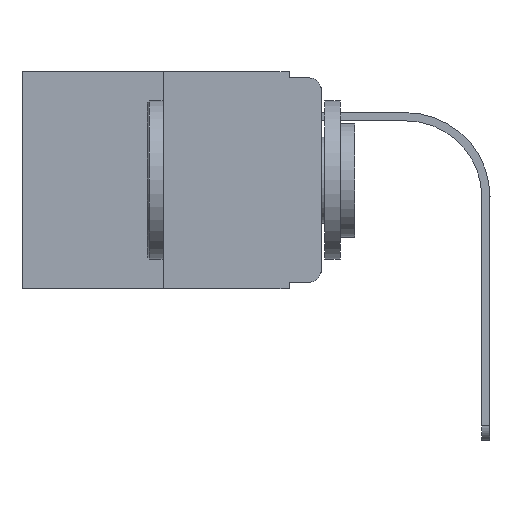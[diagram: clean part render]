
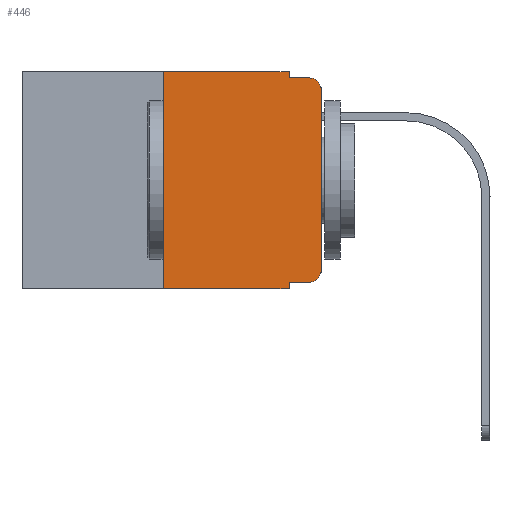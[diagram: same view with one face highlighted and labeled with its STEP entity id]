
A CAD part, left-side view. The second image highlights one B-rep face of the part: STEP entity #446.
In plain terms, the highlighted planar face has unit normal (-1, 0, 0).
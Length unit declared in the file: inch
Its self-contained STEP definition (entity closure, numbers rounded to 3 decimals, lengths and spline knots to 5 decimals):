
#70 = CIRCLE ( 'NONE', #8599, 0.02 ) ;
#167 = CARTESIAN_POINT ( 'NONE',  ( 0., 0.051, -0.01 ) ) ;
#170 = DIRECTION ( 'NONE',  ( -1., 0., 0. ) ) ;
#378 = CARTESIAN_POINT ( 'NONE',  ( 0., 0.473, 0. ) ) ;
#443 = VERTEX_POINT ( 'NONE', #7598 ) ;
#446 = ADVANCED_FACE ( 'NONE', ( #5929 ), #6590, .F. ) ;
#453 = DIRECTION ( 'NONE',  ( -1., 0., 0. ) ) ;
#575 = CARTESIAN_POINT ( 'NONE',  ( 0., 0.051, -0.343 ) ) ;
#637 = ORIENTED_EDGE ( 'NONE', *, *, #2398, .T. ) ;
#761 = EDGE_CURVE ( 'NONE', #2186, #443, #2042, .T. ) ;
#1385 = AXIS2_PLACEMENT_3D ( 'NONE', #9173, #170, #10749 ) ;
#1417 = CARTESIAN_POINT ( 'NONE',  ( 0., 0.25, -0.343 ) ) ;
#1520 = DIRECTION ( 'NONE',  ( 0., -1., 0. ) ) ;
#1544 = EDGE_CURVE ( 'NONE', #6409, #6714, #2971, .T. ) ;
#1589 = EDGE_LOOP ( 'NONE', ( #637, #8247, #5417, #9334, #9422, #5119, #8029, #5951, #1604, #4368 ) ) ;
#1604 = ORIENTED_EDGE ( 'NONE', *, *, #9402, .T. ) ;
#1634 = CARTESIAN_POINT ( 'NONE',  ( 0., 0.473, 0. ) ) ;
#2009 = CARTESIAN_POINT ( 'NONE',  ( 0., 0.051, 0. ) ) ;
#2042 = LINE ( 'NONE', #167, #7669 ) ;
#2082 = VECTOR ( 'NONE', #5662, 39.37008 ) ;
#2095 = VECTOR ( 'NONE', #1520, 39.37008 ) ;
#2110 = LINE ( 'NONE', #5325, #5553 ) ;
#2180 = LINE ( 'NONE', #3012, #2095 ) ;
#2186 = VERTEX_POINT ( 'NONE', #6053 ) ;
#2323 = CARTESIAN_POINT ( 'NONE',  ( 0., 0.051, 0. ) ) ;
#2398 = EDGE_CURVE ( 'NONE', #6714, #8966, #7943, .T. ) ;
#2554 = DIRECTION ( 'NONE',  ( 0., 0., 1. ) ) ;
#2668 = EDGE_CURVE ( 'NONE', #9132, #8607, #10073, .T. ) ;
#2971 = CIRCLE ( 'NONE', #1385, 0.02 ) ;
#3012 = CARTESIAN_POINT ( 'NONE',  ( 0., 0.473, -0.343 ) ) ;
#3018 = EDGE_CURVE ( 'NONE', #9859, #2186, #8878, .T. ) ;
#3308 = EDGE_CURVE ( 'NONE', #10294, #4684, #6876, .T. ) ;
#3467 = EDGE_CURVE ( 'NONE', #9132, #4684, #2180, .T. ) ;
#3662 = VECTOR ( 'NONE', #9560, 39.37008 ) ;
#4128 = DIRECTION ( 'NONE',  ( 0., 0., -1. ) ) ;
#4368 = ORIENTED_EDGE ( 'NONE', *, *, #1544, .T. ) ;
#4684 = VERTEX_POINT ( 'NONE', #575 ) ;
#5119 = ORIENTED_EDGE ( 'NONE', *, *, #2668, .F. ) ;
#5297 = CARTESIAN_POINT ( 'NONE',  ( 0., 0.051, 0. ) ) ;
#5325 = CARTESIAN_POINT ( 'NONE',  ( 0., 0.051, -0.333 ) ) ;
#5417 = ORIENTED_EDGE ( 'NONE', *, *, #761, .F. ) ;
#5553 = VECTOR ( 'NONE', #7751, 39.37008 ) ;
#5662 = DIRECTION ( 'NONE',  ( 0., 0., -1. ) ) ;
#5929 = FACE_OUTER_BOUND ( 'NONE', #1589, .T. ) ;
#5951 = ORIENTED_EDGE ( 'NONE', *, *, #3308, .F. ) ;
#6053 = CARTESIAN_POINT ( 'NONE',  ( 0., 0.051, -0.01 ) ) ;
#6409 = VERTEX_POINT ( 'NONE', #8992 ) ;
#6590 = PLANE ( 'NONE',  #7905 ) ;
#6611 = EDGE_CURVE ( 'NONE', #8966, #443, #70, .T. ) ;
#6714 = VERTEX_POINT ( 'NONE', #8683 ) ;
#6876 = LINE ( 'NONE', #2009, #3662 ) ;
#6948 = VECTOR ( 'NONE', #2554, 39.37008 ) ;
#6988 = VECTOR ( 'NONE', #8813, 39.37008 ) ;
#7397 = DIRECTION ( 'NONE',  ( 1., 0., 0. ) ) ;
#7598 = CARTESIAN_POINT ( 'NONE',  ( 0., 0.02, -0.01 ) ) ;
#7669 = VECTOR ( 'NONE', #8662, 39.37008 ) ;
#7751 = DIRECTION ( 'NONE',  ( 0., -1., 0. ) ) ;
#7905 = AXIS2_PLACEMENT_3D ( 'NONE', #1634, #7397, #4128 ) ;
#7908 = CARTESIAN_POINT ( 'NONE',  ( 0., 0.051, -0.333 ) ) ;
#7943 = LINE ( 'NONE', #10383, #6988 ) ;
#8029 = ORIENTED_EDGE ( 'NONE', *, *, #3467, .T. ) ;
#8247 = ORIENTED_EDGE ( 'NONE', *, *, #6611, .T. ) ;
#8316 = CARTESIAN_POINT ( 'NONE',  ( 0., 0., -0.03 ) ) ;
#8523 = DIRECTION ( 'NONE',  ( 0., 0., -1. ) ) ;
#8541 = VECTOR ( 'NONE', #9603, 39.37008 ) ;
#8599 = AXIS2_PLACEMENT_3D ( 'NONE', #10222, #453, #8523 ) ;
#8607 = VERTEX_POINT ( 'NONE', #9367 ) ;
#8662 = DIRECTION ( 'NONE',  ( 0., -1., 0. ) ) ;
#8683 = CARTESIAN_POINT ( 'NONE',  ( 0., 0., -0.313 ) ) ;
#8813 = DIRECTION ( 'NONE',  ( 0., 0., 1. ) ) ;
#8878 = LINE ( 'NONE', #2323, #2082 ) ;
#8966 = VERTEX_POINT ( 'NONE', #8316 ) ;
#8992 = CARTESIAN_POINT ( 'NONE',  ( 0., 0.02, -0.333 ) ) ;
#9132 = VERTEX_POINT ( 'NONE', #1417 ) ;
#9173 = CARTESIAN_POINT ( 'NONE',  ( 0., 0.02, -0.313 ) ) ;
#9334 = ORIENTED_EDGE ( 'NONE', *, *, #3018, .F. ) ;
#9360 = EDGE_CURVE ( 'NONE', #8607, #9859, #9498, .T. ) ;
#9367 = CARTESIAN_POINT ( 'NONE',  ( 0., 0.25, 0. ) ) ;
#9402 = EDGE_CURVE ( 'NONE', #10294, #6409, #2110, .T. ) ;
#9422 = ORIENTED_EDGE ( 'NONE', *, *, #9360, .F. ) ;
#9498 = LINE ( 'NONE', #378, #8541 ) ;
#9550 = CARTESIAN_POINT ( 'NONE',  ( 0., 0.25, 0. ) ) ;
#9560 = DIRECTION ( 'NONE',  ( 0., 0., -1. ) ) ;
#9603 = DIRECTION ( 'NONE',  ( 0., -1., 0. ) ) ;
#9859 = VERTEX_POINT ( 'NONE', #5297 ) ;
#10073 = LINE ( 'NONE', #9550, #6948 ) ;
#10222 = CARTESIAN_POINT ( 'NONE',  ( 0., 0.02, -0.03 ) ) ;
#10294 = VERTEX_POINT ( 'NONE', #7908 ) ;
#10383 = CARTESIAN_POINT ( 'NONE',  ( 0., 0., 0. ) ) ;
#10749 = DIRECTION ( 'NONE',  ( 0., 0., -1. ) ) ;
